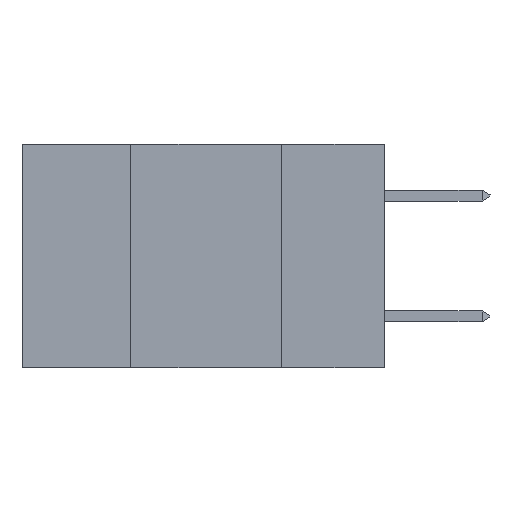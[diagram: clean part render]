
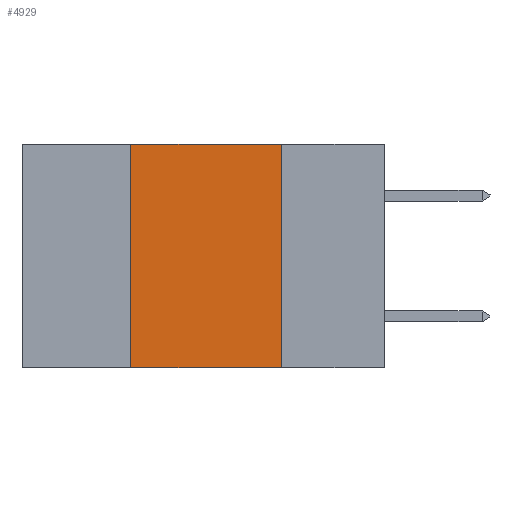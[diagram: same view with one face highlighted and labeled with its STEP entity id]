
A CAD part, left-side view. The second image highlights one B-rep face of the part: STEP entity #4929.
In plain terms, the highlighted planar face has unit normal (-1, 0, 0).
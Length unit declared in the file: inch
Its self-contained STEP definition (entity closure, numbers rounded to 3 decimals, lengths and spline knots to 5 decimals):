
#70 = EDGE_CURVE ( 'NONE', #6496, #12701, #4075, .T. ) ;
#616 = EDGE_CURVE ( 'NONE', #6496, #4597, #5742, .T. ) ;
#804 = CARTESIAN_POINT ( 'NONE',  ( 0., 0.17, -0.37 ) ) ;
#1218 = CARTESIAN_POINT ( 'NONE',  ( 0., 0.42, 0. ) ) ;
#1483 = FACE_OUTER_BOUND ( 'NONE', #8895, .T. ) ;
#1737 = CARTESIAN_POINT ( 'NONE',  ( 0., 0.6, 0. ) ) ;
#2019 = LINE ( 'NONE', #3539, #3919 ) ;
#3427 = CARTESIAN_POINT ( 'NONE',  ( 0., 0.42, -0.37 ) ) ;
#3428 = DIRECTION ( 'NONE',  ( 0., 0., 1. ) ) ;
#3539 = CARTESIAN_POINT ( 'NONE',  ( 0., 0.17, 0. ) ) ;
#3919 = VECTOR ( 'NONE', #4636, 39.37008 ) ;
#4052 = PLANE ( 'NONE',  #4293 ) ;
#4072 = DIRECTION ( 'NONE',  ( 0., -1., 0. ) ) ;
#4075 = LINE ( 'NONE', #1218, #8689 ) ;
#4293 = AXIS2_PLACEMENT_3D ( 'NONE', #11551, #7122, #6044 ) ;
#4597 = VERTEX_POINT ( 'NONE', #804 ) ;
#4636 = DIRECTION ( 'NONE',  ( 0., 0., -1. ) ) ;
#4929 = ADVANCED_FACE ( 'NONE', ( #1483 ), #4052, .F. ) ;
#5742 = LINE ( 'NONE', #7718, #14192 ) ;
#5847 = VERTEX_POINT ( 'NONE', #8526 ) ;
#6044 = DIRECTION ( 'NONE',  ( 0., 0., -1. ) ) ;
#6130 = ORIENTED_EDGE ( 'NONE', *, *, #11788, .F. ) ;
#6496 = VERTEX_POINT ( 'NONE', #3427 ) ;
#7122 = DIRECTION ( 'NONE',  ( 1., 0., 0. ) ) ;
#7718 = CARTESIAN_POINT ( 'NONE',  ( 0., 0.6, -0.37 ) ) ;
#8274 = ORIENTED_EDGE ( 'NONE', *, *, #70, .F. ) ;
#8487 = CARTESIAN_POINT ( 'NONE',  ( 0., 0.42, 0. ) ) ;
#8526 = CARTESIAN_POINT ( 'NONE',  ( 0., 0.17, 0. ) ) ;
#8683 = LINE ( 'NONE', #1737, #12282 ) ;
#8689 = VECTOR ( 'NONE', #3428, 39.37008 ) ;
#8821 = ORIENTED_EDGE ( 'NONE', *, *, #616, .T. ) ;
#8895 = EDGE_LOOP ( 'NONE', ( #6130, #13401, #8274, #8821 ) ) ;
#11551 = CARTESIAN_POINT ( 'NONE',  ( 0., 0.6, 0. ) ) ;
#11788 = EDGE_CURVE ( 'NONE', #5847, #4597, #2019, .T. ) ;
#12282 = VECTOR ( 'NONE', #12717, 39.37008 ) ;
#12538 = EDGE_CURVE ( 'NONE', #12701, #5847, #8683, .T. ) ;
#12701 = VERTEX_POINT ( 'NONE', #8487 ) ;
#12717 = DIRECTION ( 'NONE',  ( 0., -1., 0. ) ) ;
#13401 = ORIENTED_EDGE ( 'NONE', *, *, #12538, .F. ) ;
#14192 = VECTOR ( 'NONE', #4072, 39.37008 ) ;
